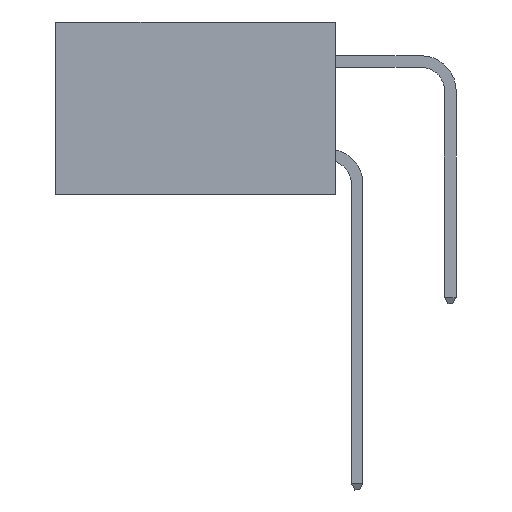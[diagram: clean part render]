
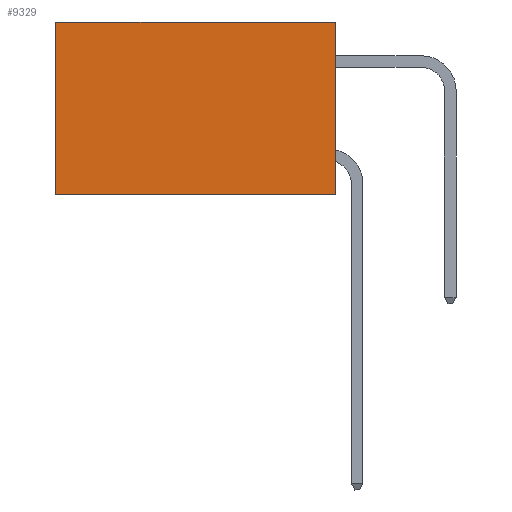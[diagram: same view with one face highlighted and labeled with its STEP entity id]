
A CAD part, left-side view. The second image highlights one B-rep face of the part: STEP entity #9329.
In plain terms, the highlighted planar face has unit normal (-1, 0, 0).
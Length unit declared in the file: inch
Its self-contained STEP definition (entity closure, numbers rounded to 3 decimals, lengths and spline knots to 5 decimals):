
#575 = DIRECTION ( 'NONE',  ( 0., 1., 0. ) ) ;
#1135 = LINE ( 'NONE', #7378, #11923 ) ;
#1157 = VERTEX_POINT ( 'NONE', #1230 ) ;
#1230 = CARTESIAN_POINT ( 'NONE',  ( 0.2875, 0., -0.37 ) ) ;
#1287 = EDGE_CURVE ( 'NONE', #7459, #12467, #13261, .T. ) ;
#1956 = CARTESIAN_POINT ( 'NONE',  ( 0.2875, 0.6, 0. ) ) ;
#2192 = CARTESIAN_POINT ( 'NONE',  ( 0.2875, 0., 0. ) ) ;
#2384 = LINE ( 'NONE', #7756, #7634 ) ;
#2563 = ORIENTED_EDGE ( 'NONE', *, *, #1287, .T. ) ;
#2661 = AXIS2_PLACEMENT_3D ( 'NONE', #2192, #4314, #11651 ) ;
#2739 = CARTESIAN_POINT ( 'NONE',  ( 0.2875, 0., 0. ) ) ;
#2809 = ORIENTED_EDGE ( 'NONE', *, *, #13185, .T. ) ;
#2947 = VECTOR ( 'NONE', #3646, 39.37008 ) ;
#3350 = DIRECTION ( 'NONE',  ( 0., 0., -1. ) ) ;
#3437 = EDGE_LOOP ( 'NONE', ( #2563, #12158, #4350, #2809 ) ) ;
#3646 = DIRECTION ( 'NONE',  ( 0., 0., -1. ) ) ;
#4314 = DIRECTION ( 'NONE',  ( 1., 0., 0. ) ) ;
#4350 = ORIENTED_EDGE ( 'NONE', *, *, #8670, .F. ) ;
#4965 = LINE ( 'NONE', #12550, #5781 ) ;
#5100 = VERTEX_POINT ( 'NONE', #2739 ) ;
#5142 = DIRECTION ( 'NONE',  ( 0., 1., 0. ) ) ;
#5347 = PLANE ( 'NONE',  #2661 ) ;
#5781 = VECTOR ( 'NONE', #3350, 39.37008 ) ;
#7378 = CARTESIAN_POINT ( 'NONE',  ( 0.2875, 0., -0.37 ) ) ;
#7459 = VERTEX_POINT ( 'NONE', #1956 ) ;
#7634 = VECTOR ( 'NONE', #575, 39.37008 ) ;
#7756 = CARTESIAN_POINT ( 'NONE',  ( 0.2875, 0., 0. ) ) ;
#8670 = EDGE_CURVE ( 'NONE', #5100, #1157, #4965, .T. ) ;
#8932 = CARTESIAN_POINT ( 'NONE',  ( 0.2875, 0.6, -0.37 ) ) ;
#9329 = ADVANCED_FACE ( 'NONE', ( #13469 ), #5347, .F. ) ;
#11651 = DIRECTION ( 'NONE',  ( 0., 0., -1. ) ) ;
#11853 = CARTESIAN_POINT ( 'NONE',  ( 0.2875, 0.6, 0. ) ) ;
#11923 = VECTOR ( 'NONE', #5142, 39.37008 ) ;
#12158 = ORIENTED_EDGE ( 'NONE', *, *, #12185, .F. ) ;
#12185 = EDGE_CURVE ( 'NONE', #1157, #12467, #1135, .T. ) ;
#12467 = VERTEX_POINT ( 'NONE', #8932 ) ;
#12550 = CARTESIAN_POINT ( 'NONE',  ( 0.2875, 0., 0. ) ) ;
#13185 = EDGE_CURVE ( 'NONE', #5100, #7459, #2384, .T. ) ;
#13261 = LINE ( 'NONE', #11853, #2947 ) ;
#13469 = FACE_OUTER_BOUND ( 'NONE', #3437, .T. ) ;
